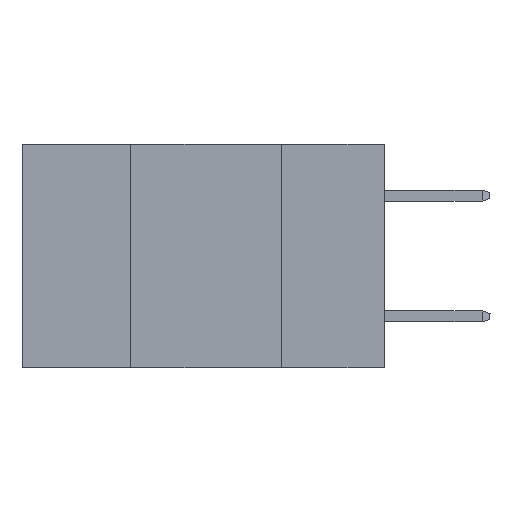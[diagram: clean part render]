
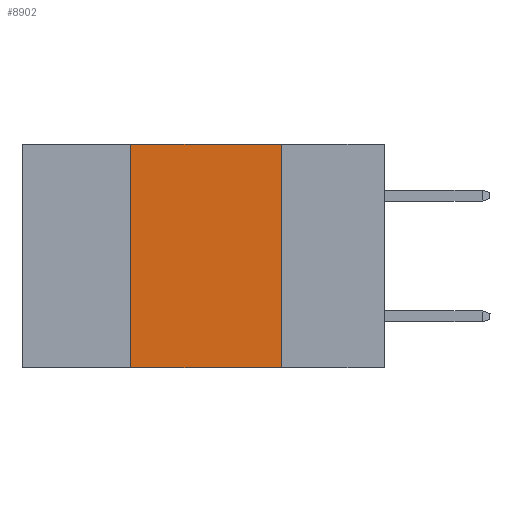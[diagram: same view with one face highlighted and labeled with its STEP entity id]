
A CAD part, left-side view. The second image highlights one B-rep face of the part: STEP entity #8902.
In plain terms, the highlighted planar face has unit normal (-1, 0, 0).
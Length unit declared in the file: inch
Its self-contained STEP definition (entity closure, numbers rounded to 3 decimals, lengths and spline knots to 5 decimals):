
#342 = VERTEX_POINT ( 'NONE', #14740 ) ;
#1258 = CARTESIAN_POINT ( 'NONE',  ( 0., 0.42, 0. ) ) ;
#2246 = EDGE_CURVE ( 'NONE', #24514, #14704, #10105, .T. ) ;
#3245 = VECTOR ( 'NONE', #19162, 39.37008 ) ;
#3377 = VECTOR ( 'NONE', #21215, 39.37008 ) ;
#3917 = CARTESIAN_POINT ( 'NONE',  ( 0., 0.42, -0.37 ) ) ;
#4857 = VECTOR ( 'NONE', #23491, 39.37008 ) ;
#6439 = ORIENTED_EDGE ( 'NONE', *, *, #7023, .F. ) ;
#6997 = CARTESIAN_POINT ( 'NONE',  ( 0., 0.42, 0. ) ) ;
#7023 = EDGE_CURVE ( 'NONE', #14704, #9347, #18993, .T. ) ;
#7591 = CARTESIAN_POINT ( 'NONE',  ( 0., 0.6, 0. ) ) ;
#7774 = AXIS2_PLACEMENT_3D ( 'NONE', #9483, #21221, #9556 ) ;
#8902 = ADVANCED_FACE ( 'NONE', ( #18397 ), #17295, .F. ) ;
#9015 = VECTOR ( 'NONE', #9684, 39.37008 ) ;
#9347 = VERTEX_POINT ( 'NONE', #24324 ) ;
#9483 = CARTESIAN_POINT ( 'NONE',  ( 0., 0.6, 0. ) ) ;
#9556 = DIRECTION ( 'NONE',  ( 0., 0., -1. ) ) ;
#9641 = LINE ( 'NONE', #19362, #9015 ) ;
#9684 = DIRECTION ( 'NONE',  ( 0., 0., -1. ) ) ;
#10105 = LINE ( 'NONE', #1258, #4857 ) ;
#11536 = EDGE_CURVE ( 'NONE', #24514, #342, #18874, .T. ) ;
#13318 = ORIENTED_EDGE ( 'NONE', *, *, #2246, .F. ) ;
#14704 = VERTEX_POINT ( 'NONE', #6997 ) ;
#14740 = CARTESIAN_POINT ( 'NONE',  ( 0., 0.17, -0.37 ) ) ;
#16157 = ORIENTED_EDGE ( 'NONE', *, *, #11536, .T. ) ;
#16678 = ORIENTED_EDGE ( 'NONE', *, *, #25164, .F. ) ;
#16742 = EDGE_LOOP ( 'NONE', ( #16678, #6439, #13318, #16157 ) ) ;
#17295 = PLANE ( 'NONE',  #7774 ) ;
#18397 = FACE_OUTER_BOUND ( 'NONE', #16742, .T. ) ;
#18874 = LINE ( 'NONE', #25048, #3245 ) ;
#18993 = LINE ( 'NONE', #7591, #3377 ) ;
#19162 = DIRECTION ( 'NONE',  ( 0., -1., 0. ) ) ;
#19362 = CARTESIAN_POINT ( 'NONE',  ( 0., 0.17, 0. ) ) ;
#21215 = DIRECTION ( 'NONE',  ( 0., -1., 0. ) ) ;
#21221 = DIRECTION ( 'NONE',  ( 1., 0., 0. ) ) ;
#23491 = DIRECTION ( 'NONE',  ( 0., 0., 1. ) ) ;
#24324 = CARTESIAN_POINT ( 'NONE',  ( 0., 0.17, 0. ) ) ;
#24514 = VERTEX_POINT ( 'NONE', #3917 ) ;
#25048 = CARTESIAN_POINT ( 'NONE',  ( 0., 0.6, -0.37 ) ) ;
#25164 = EDGE_CURVE ( 'NONE', #9347, #342, #9641, .T. ) ;
